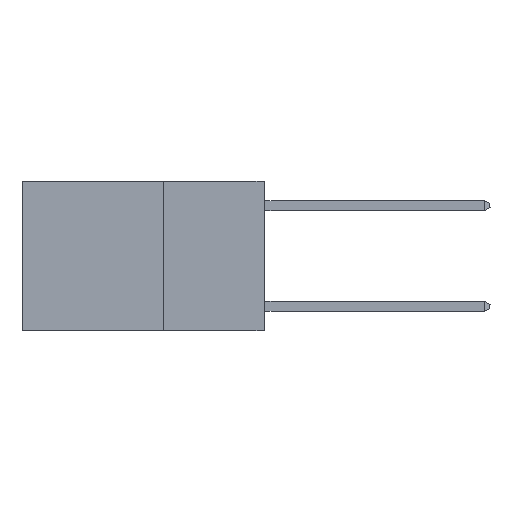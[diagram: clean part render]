
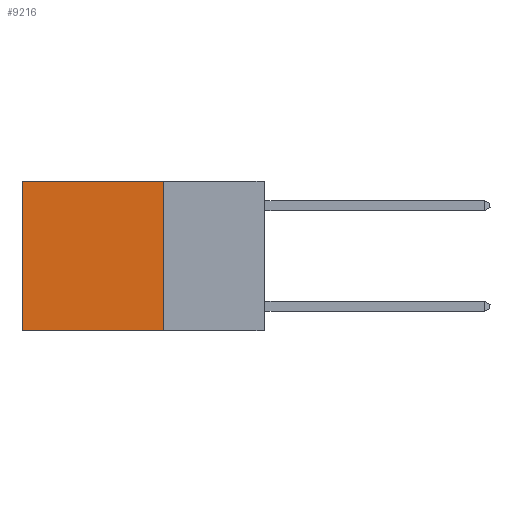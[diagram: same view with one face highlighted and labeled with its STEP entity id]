
A CAD part, left-side view. The second image highlights one B-rep face of the part: STEP entity #9216.
In plain terms, the highlighted planar face has unit normal (-1, 0, 0).
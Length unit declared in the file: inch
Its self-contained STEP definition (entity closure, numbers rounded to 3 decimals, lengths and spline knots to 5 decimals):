
#167 = CARTESIAN_POINT ( 'NONE',  ( 0.2625, 0.25, 0. ) ) ;
#743 = VERTEX_POINT ( 'NONE', #24257 ) ;
#2146 = VECTOR ( 'NONE', #26194, 39.37008 ) ;
#2289 = VERTEX_POINT ( 'NONE', #23931 ) ;
#3628 = AXIS2_PLACEMENT_3D ( 'NONE', #13988, #18485, #22992 ) ;
#4403 = LINE ( 'NONE', #23877, #17698 ) ;
#7921 = VERTEX_POINT ( 'NONE', #167 ) ;
#8025 = FACE_OUTER_BOUND ( 'NONE', #21427, .T. ) ;
#8875 = EDGE_CURVE ( 'NONE', #743, #10763, #20802, .T. ) ;
#9216 = ADVANCED_FACE ( 'NONE', ( #8025 ), #14532, .F. ) ;
#9440 = CARTESIAN_POINT ( 'NONE',  ( 0.2625, 0.25, 0. ) ) ;
#10763 = VERTEX_POINT ( 'NONE', #24887 ) ;
#11574 = LINE ( 'NONE', #9440, #19471 ) ;
#12052 = CARTESIAN_POINT ( 'NONE',  ( 0.2625, 0.25, -0.37 ) ) ;
#12106 = EDGE_CURVE ( 'NONE', #2289, #10763, #4403, .T. ) ;
#13202 = LINE ( 'NONE', #14311, #2146 ) ;
#13649 = ORIENTED_EDGE ( 'NONE', *, *, #24735, .F. ) ;
#13988 = CARTESIAN_POINT ( 'NONE',  ( 0.2625, 0.25, 0. ) ) ;
#14311 = CARTESIAN_POINT ( 'NONE',  ( 0.2625, 0.25, 0. ) ) ;
#14532 = PLANE ( 'NONE',  #3628 ) ;
#14928 = ORIENTED_EDGE ( 'NONE', *, *, #8875, .F. ) ;
#15330 = VECTOR ( 'NONE', #20391, 39.37008 ) ;
#17698 = VECTOR ( 'NONE', #21621, 39.37008 ) ;
#18049 = DIRECTION ( 'NONE',  ( 0., 0., -1. ) ) ;
#18149 = ORIENTED_EDGE ( 'NONE', *, *, #12106, .T. ) ;
#18485 = DIRECTION ( 'NONE',  ( 1., 0., 0. ) ) ;
#19334 = EDGE_CURVE ( 'NONE', #7921, #2289, #13202, .T. ) ;
#19471 = VECTOR ( 'NONE', #18049, 39.37008 ) ;
#19758 = ORIENTED_EDGE ( 'NONE', *, *, #19334, .T. ) ;
#20391 = DIRECTION ( 'NONE',  ( 0., 1., 0. ) ) ;
#20802 = LINE ( 'NONE', #12052, #15330 ) ;
#21427 = EDGE_LOOP ( 'NONE', ( #18149, #14928, #13649, #19758 ) ) ;
#21621 = DIRECTION ( 'NONE',  ( 0., 0., -1. ) ) ;
#22992 = DIRECTION ( 'NONE',  ( 0., 0., -1. ) ) ;
#23877 = CARTESIAN_POINT ( 'NONE',  ( 0.2625, 0.6, 0. ) ) ;
#23931 = CARTESIAN_POINT ( 'NONE',  ( 0.2625, 0.6, 0. ) ) ;
#24257 = CARTESIAN_POINT ( 'NONE',  ( 0.2625, 0.25, -0.37 ) ) ;
#24735 = EDGE_CURVE ( 'NONE', #7921, #743, #11574, .T. ) ;
#24887 = CARTESIAN_POINT ( 'NONE',  ( 0.2625, 0.6, -0.37 ) ) ;
#26194 = DIRECTION ( 'NONE',  ( 0., 1., 0. ) ) ;
